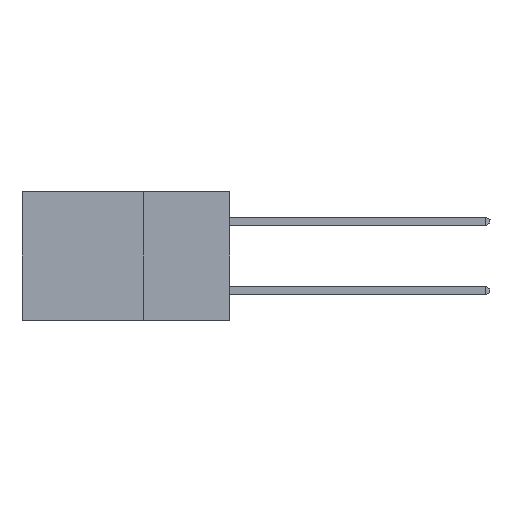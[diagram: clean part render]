
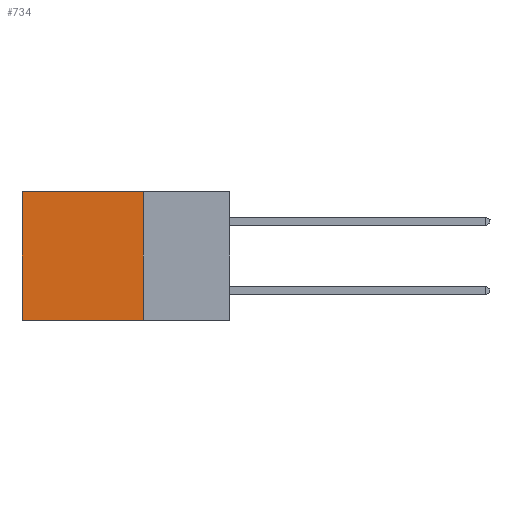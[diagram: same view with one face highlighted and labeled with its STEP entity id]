
A CAD part, left-side view. The second image highlights one B-rep face of the part: STEP entity #734.
In plain terms, the highlighted planar face has unit normal (-1, 0, 0).
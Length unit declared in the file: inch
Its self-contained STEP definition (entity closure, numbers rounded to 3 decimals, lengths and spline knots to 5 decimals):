
#734 = ADVANCED_FACE ( 'NONE', ( #12451 ), #19917, .F. ) ;
#966 = EDGE_LOOP ( 'NONE', ( #5915, #10307, #16743, #12106 ) ) ;
#977 = DIRECTION ( 'NONE',  ( 0., 0., -1. ) ) ;
#1466 = VERTEX_POINT ( 'NONE', #21424 ) ;
#2835 = CARTESIAN_POINT ( 'NONE',  ( 0.298, 0.25, 0. ) ) ;
#4726 = CARTESIAN_POINT ( 'NONE',  ( 0.298, 0.6, 0. ) ) ;
#5915 = ORIENTED_EDGE ( 'NONE', *, *, #25509, .T. ) ;
#6659 = VERTEX_POINT ( 'NONE', #21804 ) ;
#9054 = LINE ( 'NONE', #20101, #13055 ) ;
#10307 = ORIENTED_EDGE ( 'NONE', *, *, #15239, .F. ) ;
#12106 = ORIENTED_EDGE ( 'NONE', *, *, #16400, .T. ) ;
#12451 = FACE_OUTER_BOUND ( 'NONE', #966, .T. ) ;
#13055 = VECTOR ( 'NONE', #21953, 39.37008 ) ;
#13356 = DIRECTION ( 'NONE',  ( 0., 1., 0. ) ) ;
#13367 = EDGE_CURVE ( 'NONE', #6659, #1466, #24726, .T. ) ;
#13495 = VECTOR ( 'NONE', #25448, 39.37008 ) ;
#13721 = CARTESIAN_POINT ( 'NONE',  ( 0.298, 0.25, 0. ) ) ;
#14165 = VECTOR ( 'NONE', #25984, 39.37008 ) ;
#14958 = VERTEX_POINT ( 'NONE', #16350 ) ;
#15239 = EDGE_CURVE ( 'NONE', #1466, #14958, #19747, .T. ) ;
#16350 = CARTESIAN_POINT ( 'NONE',  ( 0.298, 0.6, -0.37 ) ) ;
#16400 = EDGE_CURVE ( 'NONE', #6659, #16707, #9054, .T. ) ;
#16408 = VECTOR ( 'NONE', #13356, 39.37008 ) ;
#16707 = VERTEX_POINT ( 'NONE', #27279 ) ;
#16743 = ORIENTED_EDGE ( 'NONE', *, *, #13367, .F. ) ;
#16818 = LINE ( 'NONE', #4726, #13495 ) ;
#18022 = AXIS2_PLACEMENT_3D ( 'NONE', #13721, #26173, #977 ) ;
#19747 = LINE ( 'NONE', #26085, #16408 ) ;
#19917 = PLANE ( 'NONE',  #18022 ) ;
#20101 = CARTESIAN_POINT ( 'NONE',  ( 0.298, 0.25, 0. ) ) ;
#21424 = CARTESIAN_POINT ( 'NONE',  ( 0.298, 0.25, -0.37 ) ) ;
#21804 = CARTESIAN_POINT ( 'NONE',  ( 0.298, 0.25, 0. ) ) ;
#21953 = DIRECTION ( 'NONE',  ( 0., 1., 0. ) ) ;
#24726 = LINE ( 'NONE', #2835, #14165 ) ;
#25448 = DIRECTION ( 'NONE',  ( 0., 0., -1. ) ) ;
#25509 = EDGE_CURVE ( 'NONE', #16707, #14958, #16818, .T. ) ;
#25984 = DIRECTION ( 'NONE',  ( 0., 0., -1. ) ) ;
#26085 = CARTESIAN_POINT ( 'NONE',  ( 0.298, 0.25, -0.37 ) ) ;
#26173 = DIRECTION ( 'NONE',  ( 1., 0., 0. ) ) ;
#27279 = CARTESIAN_POINT ( 'NONE',  ( 0.298, 0.6, 0. ) ) ;
